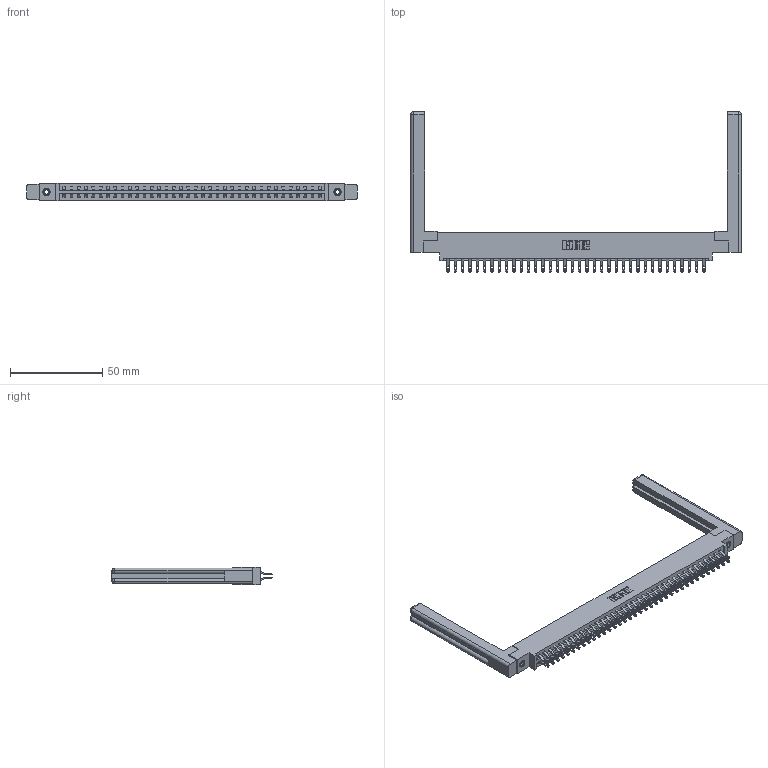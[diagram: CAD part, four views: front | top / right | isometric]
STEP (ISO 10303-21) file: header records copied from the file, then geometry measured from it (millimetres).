
FILE_DESCRIPTION (( 'STEP AP203' ), '1' );
FILE_NAME ('387-072-555-858.STEP', '2019-10-22T00:26:59', ( '' ), ( '' ), 'SwSTEP 2.0', 'SolidWorks 2016', '' );
FILE_SCHEMA (( 'CONFIG_CONTROL_DESIGN' ));
Length unit declared in the file: inch
Products named in the file (5): 387-072-555-858; 337 Part_0.170 Offset - 0.156 Dia-TI; 345-292-001_555 Tail; 307-220-058; 345-250-001_345-250-001-102
Assembly tree (77 placements, depth 2):
  387-072-555-858
    337 Part_0.170 Offset - 0.156 Dia-TI
    345-292-001_555 Tail  x72
    345-250-001_345-250-001-102  x2
    307-220-058  x2
Bounding box: 179.27 x 86.87 x 9.4 mm (x, y, z)
Volume: 26047 mm3; surface area: 27255.1 mm2
Topology: 77 solids, 77 shells, 4580 faces, 14285 edges, 9510 vertices
Faces by surface type: plane 2750, cylinder 1806, cone 12, torus 12
Entity records: 31780 total; most frequent: CARTESIAN_POINT 5403, ORIENTED_EDGE 5248, DIRECTION 4592, EDGE_CURVE 2624, VECTOR 2428, LINE 2428, VERTEX_POINT 1742, AXIS2_PLACEMENT_3D 1082
